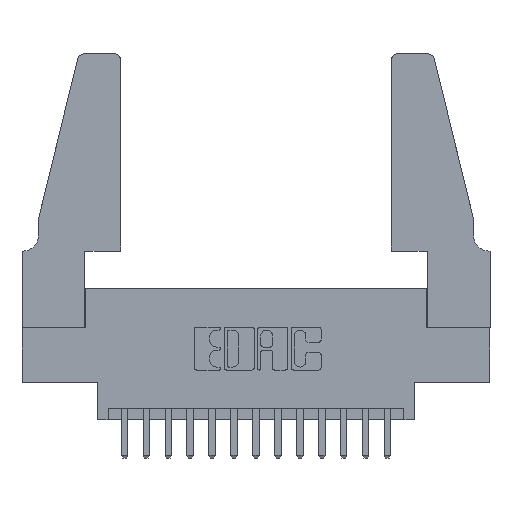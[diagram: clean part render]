
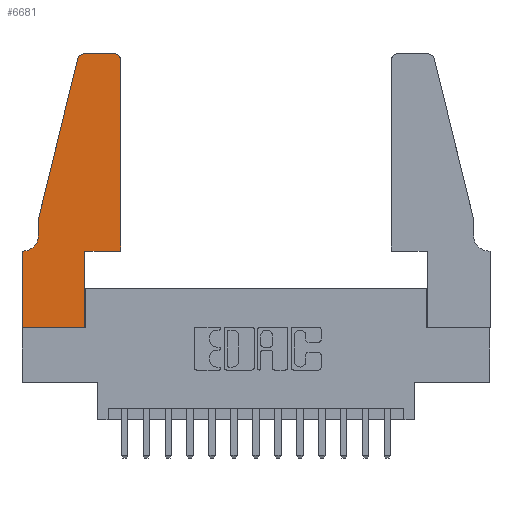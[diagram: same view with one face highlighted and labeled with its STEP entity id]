
A CAD part, top view. The second image highlights one B-rep face of the part: STEP entity #6681.
In plain terms, the highlighted planar face has unit normal (0, 0, 1).
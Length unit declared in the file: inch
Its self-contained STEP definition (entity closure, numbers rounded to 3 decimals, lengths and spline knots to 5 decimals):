
#125 = AXIS2_PLACEMENT_3D ( 'NONE', #15929, #8347, #641 ) ;
#222 = CARTESIAN_POINT ( 'NONE',  ( 0., 0.35, 0.37 ) ) ;
#333 = DIRECTION ( 'NONE',  ( 0., -1., 0. ) ) ;
#578 = ORIENTED_EDGE ( 'NONE', *, *, #14280, .T. ) ;
#641 = DIRECTION ( 'NONE',  ( -1., 0., 0. ) ) ;
#653 = DIRECTION ( 'NONE',  ( 1., 0., 0. ) ) ;
#723 = ORIENTED_EDGE ( 'NONE', *, *, #1199, .T. ) ;
#861 = ORIENTED_EDGE ( 'NONE', *, *, #10149, .T. ) ;
#887 = CARTESIAN_POINT ( 'NONE',  ( 0.2865, 0.35, 0.37 ) ) ;
#1199 = EDGE_CURVE ( 'NONE', #14241, #14190, #6173, .T. ) ;
#1315 = ORIENTED_EDGE ( 'NONE', *, *, #1438, .T. ) ;
#1438 = EDGE_CURVE ( 'NONE', #4833, #9870, #16097, .T. ) ;
#1557 = ORIENTED_EDGE ( 'NONE', *, *, #14703, .T. ) ;
#1589 = AXIS2_PLACEMENT_3D ( 'NONE', #3624, #12572, #4942 ) ;
#1729 = VECTOR ( 'NONE', #12118, 39.37008 ) ;
#1830 = CARTESIAN_POINT ( 'NONE',  ( 0.0755, 0.42, 0.37 ) ) ;
#1897 = ORIENTED_EDGE ( 'NONE', *, *, #5849, .T. ) ;
#1988 = CARTESIAN_POINT ( 'NONE',  ( 0.25487, 1.22718, 0.37 ) ) ;
#2045 = ORIENTED_EDGE ( 'NONE', *, *, #8919, .T. ) ;
#2424 = CARTESIAN_POINT ( 'NONE',  ( 0.4205, 1.25, 0.37 ) ) ;
#2432 = ORIENTED_EDGE ( 'NONE', *, *, #16516, .T. ) ;
#2448 = CARTESIAN_POINT ( 'NONE',  ( 0., 0.35, 0.37 ) ) ;
#2511 = CARTESIAN_POINT ( 'NONE',  ( 0.0755, 0.5, 0.37 ) ) ;
#2651 = EDGE_CURVE ( 'NONE', #12905, #16435, #4913, .T. ) ;
#2740 = VECTOR ( 'NONE', #9802, 39.37008 ) ;
#2902 = CARTESIAN_POINT ( 'NONE',  ( 0., 0., 0.37 ) ) ;
#2950 = DIRECTION ( 'NONE',  ( -1., 0., 0. ) ) ;
#3048 = LINE ( 'NONE', #7640, #12877 ) ;
#3172 = CARTESIAN_POINT ( 'NONE',  ( 0.0755, 0.5, 0.37 ) ) ;
#3345 = ORIENTED_EDGE ( 'NONE', *, *, #4072, .T. ) ;
#3624 = CARTESIAN_POINT ( 'NONE',  ( 0.284, 1.22, 0.37 ) ) ;
#3738 = DIRECTION ( 'NONE',  ( 0., 0., 1. ) ) ;
#4072 = EDGE_CURVE ( 'NONE', #14190, #14497, #7074, .T. ) ;
#4211 = DIRECTION ( 'NONE',  ( 0., 1., 0. ) ) ;
#4833 = VERTEX_POINT ( 'NONE', #13559 ) ;
#4913 = LINE ( 'NONE', #7189, #8328 ) ;
#4942 = DIRECTION ( 'NONE',  ( 1., 0., 0. ) ) ;
#5476 = VERTEX_POINT ( 'NONE', #16076 ) ;
#5684 = EDGE_CURVE ( 'NONE', #5476, #14241, #3048, .T. ) ;
#5692 = VERTEX_POINT ( 'NONE', #2511 ) ;
#5849 = EDGE_CURVE ( 'NONE', #9870, #16187, #10079, .T. ) ;
#6043 = VERTEX_POINT ( 'NONE', #1988 ) ;
#6173 = LINE ( 'NONE', #13152, #2740 ) ;
#6681 = ADVANCED_FACE ( 'NONE', ( #8260 ), #10136, .T. ) ;
#6683 = VECTOR ( 'NONE', #10570, 39.37008 ) ;
#6734 = CARTESIAN_POINT ( 'NONE',  ( 0.2605, 1.25, 0.37 ) ) ;
#6738 = LINE ( 'NONE', #8106, #16463 ) ;
#6981 = CIRCLE ( 'NONE', #1589, 0.03 ) ;
#7040 = EDGE_CURVE ( 'NONE', #10771, #12905, #8651, .T. ) ;
#7069 = CARTESIAN_POINT ( 'NONE',  ( 0.4505, 0.35, 0.37 ) ) ;
#7074 = LINE ( 'NONE', #7069, #10853 ) ;
#7100 = DIRECTION ( 'NONE',  ( 0., 0., 1. ) ) ;
#7135 = VECTOR ( 'NONE', #333, 39.37008 ) ;
#7189 = CARTESIAN_POINT ( 'NONE',  ( 0.0755, 0.35, 0.37 ) ) ;
#7640 = CARTESIAN_POINT ( 'NONE',  ( 0., 0., 0.37 ) ) ;
#7859 = ORIENTED_EDGE ( 'NONE', *, *, #7040, .T. ) ;
#8106 = CARTESIAN_POINT ( 'NONE',  ( 0.4505, 0.35, 0.37 ) ) ;
#8118 = ORIENTED_EDGE ( 'NONE', *, *, #2651, .T. ) ;
#8195 = AXIS2_PLACEMENT_3D ( 'NONE', #8279, #7100, #10018 ) ;
#8260 = FACE_OUTER_BOUND ( 'NONE', #9747, .T. ) ;
#8279 = CARTESIAN_POINT ( 'NONE',  ( 0.4205, 1.22, 0.37 ) ) ;
#8328 = VECTOR ( 'NONE', #2950, 39.37008 ) ;
#8347 = DIRECTION ( 'NONE',  ( 0., 0., -1. ) ) ;
#8651 = CIRCLE ( 'NONE', #125, 0.07 ) ;
#8919 = EDGE_CURVE ( 'NONE', #6043, #5692, #15337, .T. ) ;
#9747 = EDGE_LOOP ( 'NONE', ( #1897, #578, #2045, #1557, #7859, #8118, #2432, #14073, #723, #3345, #861, #1315 ) ) ;
#9802 = DIRECTION ( 'NONE',  ( 0., 1., 0. ) ) ;
#9870 = VERTEX_POINT ( 'NONE', #2424 ) ;
#9920 = CARTESIAN_POINT ( 'NONE',  ( 0.2865, 0., 0.37 ) ) ;
#9959 = CARTESIAN_POINT ( 'NONE',  ( 0.0755, 0.5, 0.37 ) ) ;
#10018 = DIRECTION ( 'NONE',  ( 1., 0., 0. ) ) ;
#10079 = LINE ( 'NONE', #6734, #6683 ) ;
#10136 = PLANE ( 'NONE',  #12781 ) ;
#10149 = EDGE_CURVE ( 'NONE', #14497, #4833, #6738, .T. ) ;
#10516 = CARTESIAN_POINT ( 'NONE',  ( 0.4505, 0.35, 0.37 ) ) ;
#10570 = DIRECTION ( 'NONE',  ( -1., 0., 0. ) ) ;
#10576 = VECTOR ( 'NONE', #16270, 39.37008 ) ;
#10771 = VERTEX_POINT ( 'NONE', #1830 ) ;
#10853 = VECTOR ( 'NONE', #653, 39.37008 ) ;
#11176 = CARTESIAN_POINT ( 'NONE',  ( 0.0055, 0.35, 0.37 ) ) ;
#12118 = DIRECTION ( 'NONE',  ( -0.239, -0.971, 0. ) ) ;
#12572 = DIRECTION ( 'NONE',  ( 0., 0., 1. ) ) ;
#12694 = DIRECTION ( 'NONE',  ( 1., 0., 0. ) ) ;
#12781 = AXIS2_PLACEMENT_3D ( 'NONE', #2448, #3738, #12694 ) ;
#12877 = VECTOR ( 'NONE', #15256, 39.37008 ) ;
#12905 = VERTEX_POINT ( 'NONE', #11176 ) ;
#13152 = CARTESIAN_POINT ( 'NONE',  ( 0.2865, 0.35, 0.37 ) ) ;
#13559 = CARTESIAN_POINT ( 'NONE',  ( 0.4505, 1.22, 0.37 ) ) ;
#13565 = LINE ( 'NONE', #9959, #10576 ) ;
#14073 = ORIENTED_EDGE ( 'NONE', *, *, #5684, .T. ) ;
#14190 = VERTEX_POINT ( 'NONE', #887 ) ;
#14241 = VERTEX_POINT ( 'NONE', #9920 ) ;
#14280 = EDGE_CURVE ( 'NONE', #16187, #6043, #6981, .T. ) ;
#14497 = VERTEX_POINT ( 'NONE', #10516 ) ;
#14703 = EDGE_CURVE ( 'NONE', #5692, #10771, #13565, .T. ) ;
#15092 = CARTESIAN_POINT ( 'NONE',  ( 0.284, 1.25, 0.37 ) ) ;
#15256 = DIRECTION ( 'NONE',  ( 1., 0., 0. ) ) ;
#15337 = LINE ( 'NONE', #3172, #1729 ) ;
#15929 = CARTESIAN_POINT ( 'NONE',  ( 0.0055, 0.42, 0.37 ) ) ;
#16076 = CARTESIAN_POINT ( 'NONE',  ( 0., 0., 0.37 ) ) ;
#16097 = CIRCLE ( 'NONE', #8195, 0.03 ) ;
#16187 = VERTEX_POINT ( 'NONE', #15092 ) ;
#16270 = DIRECTION ( 'NONE',  ( 0., -1., 0. ) ) ;
#16435 = VERTEX_POINT ( 'NONE', #222 ) ;
#16458 = LINE ( 'NONE', #2902, #7135 ) ;
#16463 = VECTOR ( 'NONE', #4211, 39.37008 ) ;
#16516 = EDGE_CURVE ( 'NONE', #16435, #5476, #16458, .T. ) ;
